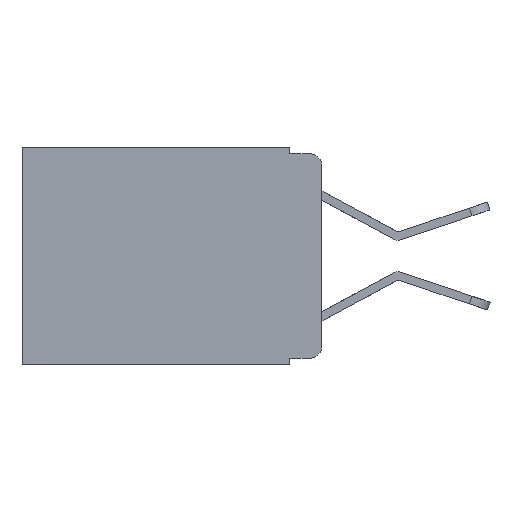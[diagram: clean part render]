
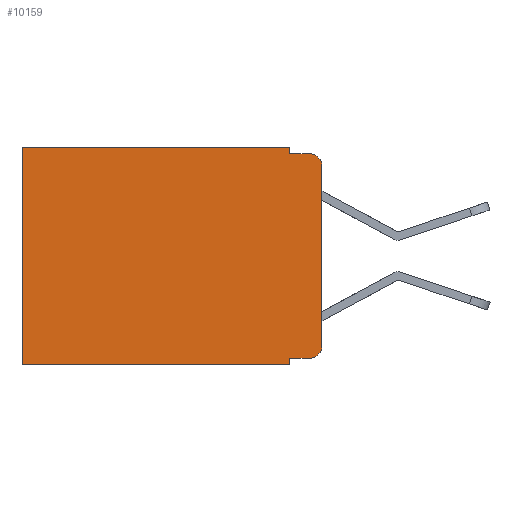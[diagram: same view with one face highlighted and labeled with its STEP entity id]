
A CAD part, left-side view. The second image highlights one B-rep face of the part: STEP entity #10159.
In plain terms, the highlighted planar face has unit normal (-1, 0, 0).
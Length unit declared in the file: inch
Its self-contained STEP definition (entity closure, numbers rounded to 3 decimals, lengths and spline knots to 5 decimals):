
#312 = DIRECTION ( 'NONE',  ( 0., -1., 0. ) ) ;
#331 = CARTESIAN_POINT ( 'NONE',  ( 0.298, 0.051, -0.343 ) ) ;
#408 = VERTEX_POINT ( 'NONE', #5734 ) ;
#431 = VERTEX_POINT ( 'NONE', #4558 ) ;
#630 = DIRECTION ( 'NONE',  ( 0., 1., 0. ) ) ;
#753 = VERTEX_POINT ( 'NONE', #13200 ) ;
#929 = EDGE_LOOP ( 'NONE', ( #11146, #14536, #6232, #1475, #6076, #7855, #10248, #5797, #13954, #11803 ) ) ;
#1247 = CIRCLE ( 'NONE', #9938, 0.02 ) ;
#1366 = CARTESIAN_POINT ( 'NONE',  ( 0.298, 0.051, -0.01 ) ) ;
#1434 = CARTESIAN_POINT ( 'NONE',  ( 0.298, 0.02, -0.03 ) ) ;
#1453 = VECTOR ( 'NONE', #8118, 39.37008 ) ;
#1475 = ORIENTED_EDGE ( 'NONE', *, *, #4229, .F. ) ;
#1901 = VERTEX_POINT ( 'NONE', #8108 ) ;
#1955 = EDGE_CURVE ( 'NONE', #9787, #431, #1247, .T. ) ;
#2135 = AXIS2_PLACEMENT_3D ( 'NONE', #8794, #11219, #9967 ) ;
#2524 = EDGE_CURVE ( 'NONE', #12491, #1901, #3896, .T. ) ;
#2548 = LINE ( 'NONE', #6051, #6068 ) ;
#2770 = PLANE ( 'NONE',  #2135 ) ;
#3219 = CARTESIAN_POINT ( 'NONE',  ( 0.298, 0.051, 0. ) ) ;
#3428 = CARTESIAN_POINT ( 'NONE',  ( 0.298, 0., -0.03 ) ) ;
#3896 = CIRCLE ( 'NONE', #9418, 0.02 ) ;
#3961 = LINE ( 'NONE', #8750, #9135 ) ;
#4229 = EDGE_CURVE ( 'NONE', #753, #8068, #10251, .T. ) ;
#4390 = CARTESIAN_POINT ( 'NONE',  ( 0.298, 0.02, -0.313 ) ) ;
#4558 = CARTESIAN_POINT ( 'NONE',  ( 0.298, 0.02, -0.01 ) ) ;
#4624 = DIRECTION ( 'NONE',  ( 0., 0., -1. ) ) ;
#4942 = LINE ( 'NONE', #6031, #6288 ) ;
#5260 = DIRECTION ( 'NONE',  ( 0., 0., -1. ) ) ;
#5409 = LINE ( 'NONE', #14659, #10848 ) ;
#5433 = VECTOR ( 'NONE', #6431, 39.37008 ) ;
#5734 = CARTESIAN_POINT ( 'NONE',  ( 0.298, 0.473, 0. ) ) ;
#5797 = ORIENTED_EDGE ( 'NONE', *, *, #10887, .F. ) ;
#6031 = CARTESIAN_POINT ( 'NONE',  ( 0.298, 0., 0. ) ) ;
#6051 = CARTESIAN_POINT ( 'NONE',  ( 0.298, 0.051, -0.333 ) ) ;
#6068 = VECTOR ( 'NONE', #312, 39.37008 ) ;
#6076 = ORIENTED_EDGE ( 'NONE', *, *, #15208, .T. ) ;
#6160 = DIRECTION ( 'NONE',  ( 0., 0., -1. ) ) ;
#6194 = DIRECTION ( 'NONE',  ( 0., 0., -1. ) ) ;
#6232 = ORIENTED_EDGE ( 'NONE', *, *, #13536, .F. ) ;
#6277 = FACE_OUTER_BOUND ( 'NONE', #929, .T. ) ;
#6288 = VECTOR ( 'NONE', #6194, 39.37008 ) ;
#6389 = DIRECTION ( 'NONE',  ( -1., 0., 0. ) ) ;
#6431 = DIRECTION ( 'NONE',  ( 0., 1., 0. ) ) ;
#6822 = VECTOR ( 'NONE', #15334, 39.37008 ) ;
#7056 = CARTESIAN_POINT ( 'NONE',  ( 0.298, 0.051, -0.333 ) ) ;
#7184 = VECTOR ( 'NONE', #630, 39.37008 ) ;
#7221 = EDGE_CURVE ( 'NONE', #15351, #12491, #2548, .T. ) ;
#7570 = EDGE_CURVE ( 'NONE', #9787, #1901, #4942, .T. ) ;
#7627 = VERTEX_POINT ( 'NONE', #331 ) ;
#7855 = ORIENTED_EDGE ( 'NONE', *, *, #10166, .T. ) ;
#8040 = CARTESIAN_POINT ( 'NONE',  ( 0.298, 0.051, -0.01 ) ) ;
#8068 = VERTEX_POINT ( 'NONE', #1366 ) ;
#8108 = CARTESIAN_POINT ( 'NONE',  ( 0.298, 0., -0.313 ) ) ;
#8118 = DIRECTION ( 'NONE',  ( 0., -1., 0. ) ) ;
#8670 = DIRECTION ( 'NONE',  ( 0., 0., -1. ) ) ;
#8750 = CARTESIAN_POINT ( 'NONE',  ( 0.298, 0.051, 0. ) ) ;
#8787 = CARTESIAN_POINT ( 'NONE',  ( 0.298, 0., 0. ) ) ;
#8794 = CARTESIAN_POINT ( 'NONE',  ( 0.298, 0., 0. ) ) ;
#9135 = VECTOR ( 'NONE', #8670, 39.37008 ) ;
#9418 = AXIS2_PLACEMENT_3D ( 'NONE', #4390, #12779, #4624 ) ;
#9532 = CARTESIAN_POINT ( 'NONE',  ( 0.298, 0.02, -0.333 ) ) ;
#9787 = VERTEX_POINT ( 'NONE', #3428 ) ;
#9938 = AXIS2_PLACEMENT_3D ( 'NONE', #1434, #6389, #6160 ) ;
#9967 = DIRECTION ( 'NONE',  ( 0., 0., -1. ) ) ;
#10159 = ADVANCED_FACE ( 'NONE', ( #6277 ), #2770, .F. ) ;
#10166 = EDGE_CURVE ( 'NONE', #408, #11161, #5409, .T. ) ;
#10248 = ORIENTED_EDGE ( 'NONE', *, *, #12669, .F. ) ;
#10251 = LINE ( 'NONE', #3219, #6822 ) ;
#10264 = LINE ( 'NONE', #8787, #5433 ) ;
#10848 = VECTOR ( 'NONE', #5260, 39.37008 ) ;
#10887 = EDGE_CURVE ( 'NONE', #15351, #7627, #3961, .T. ) ;
#10994 = CARTESIAN_POINT ( 'NONE',  ( 0.298, 0., -0.343 ) ) ;
#11146 = ORIENTED_EDGE ( 'NONE', *, *, #7570, .F. ) ;
#11161 = VERTEX_POINT ( 'NONE', #11720 ) ;
#11219 = DIRECTION ( 'NONE',  ( 1., 0., 0. ) ) ;
#11720 = CARTESIAN_POINT ( 'NONE',  ( 0.298, 0.473, -0.343 ) ) ;
#11803 = ORIENTED_EDGE ( 'NONE', *, *, #2524, .T. ) ;
#12411 = LINE ( 'NONE', #10994, #7184 ) ;
#12491 = VERTEX_POINT ( 'NONE', #9532 ) ;
#12669 = EDGE_CURVE ( 'NONE', #7627, #11161, #12411, .T. ) ;
#12779 = DIRECTION ( 'NONE',  ( -1., 0., 0. ) ) ;
#13200 = CARTESIAN_POINT ( 'NONE',  ( 0.298, 0.051, 0. ) ) ;
#13536 = EDGE_CURVE ( 'NONE', #8068, #431, #15388, .T. ) ;
#13954 = ORIENTED_EDGE ( 'NONE', *, *, #7221, .T. ) ;
#14536 = ORIENTED_EDGE ( 'NONE', *, *, #1955, .T. ) ;
#14659 = CARTESIAN_POINT ( 'NONE',  ( 0.298, 0.473, 0. ) ) ;
#15208 = EDGE_CURVE ( 'NONE', #753, #408, #10264, .T. ) ;
#15334 = DIRECTION ( 'NONE',  ( 0., 0., -1. ) ) ;
#15351 = VERTEX_POINT ( 'NONE', #7056 ) ;
#15388 = LINE ( 'NONE', #8040, #1453 ) ;
